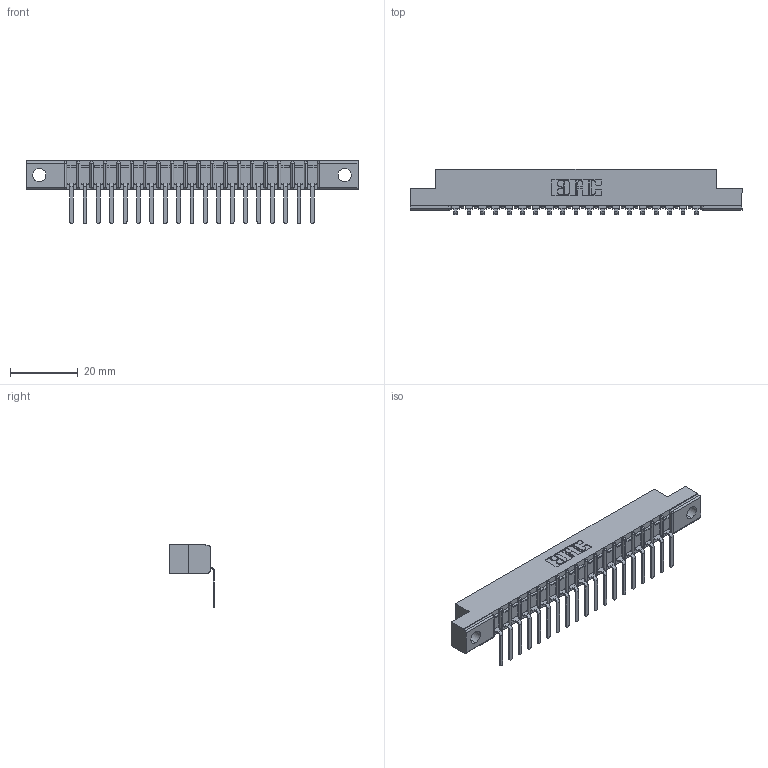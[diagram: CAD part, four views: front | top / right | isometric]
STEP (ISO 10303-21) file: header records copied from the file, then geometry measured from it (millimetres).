
FILE_DESCRIPTION (( 'STEP AP203' ), '1' );
FILE_NAME ('307-019-557-104.STEP', '2019-09-04T22:52:21', ( '' ), ( '' ), 'SwSTEP 2.0', 'SolidWorks 2016', '' );
FILE_SCHEMA (( 'CONFIG_CONTROL_DESIGN' ));
Length unit declared in the file: inch
Products named in the file (3): 307-290-002_557; 307-019-557-104; 307 Part_.156 Dia Mounting Holes
Assembly tree (20 placements, depth 2):
  307-019-557-104
    307 Part_.156 Dia Mounting Holes
    307-290-002_557  x19
Bounding box: 98.3 x 13.32 x 18.67 mm (x, y, z)
Volume: 6433.2 mm3; surface area: 11738.2 mm2
Topology: 20 solids, 20 shells, 1634 faces, 4995 edges, 3274 vertices
Faces by surface type: plane 977, cylinder 617, sphere 40
Entity records: 20396 total; most frequent: CARTESIAN_POINT 3442, ORIENTED_EDGE 3430, DIRECTION 3347, EDGE_CURVE 1715, LINE 1309, VECTOR 1309, VERTEX_POINT 1114, AXIS2_PLACEMENT_3D 1019
